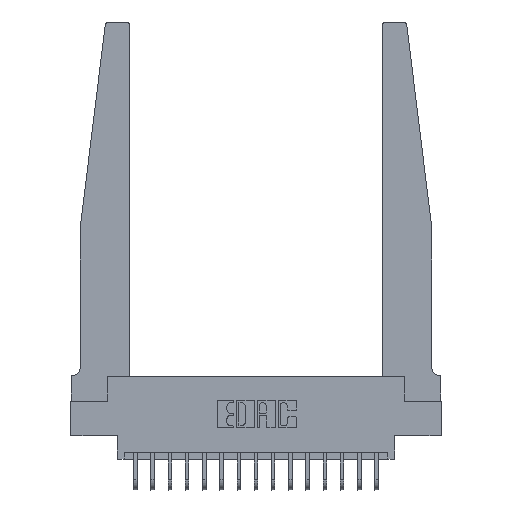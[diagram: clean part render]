
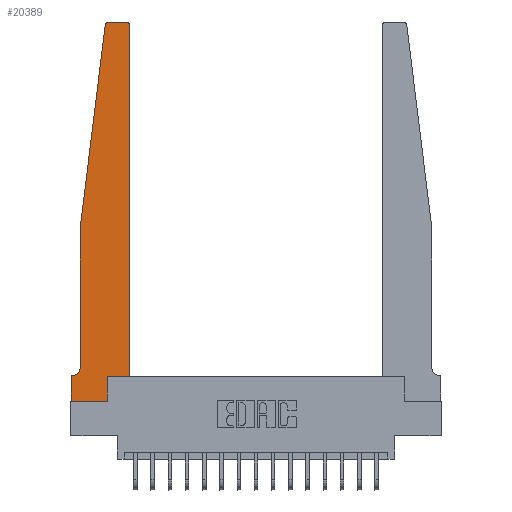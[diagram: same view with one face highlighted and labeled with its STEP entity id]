
A CAD part, top view. The second image highlights one B-rep face of the part: STEP entity #20389.
In plain terms, the highlighted planar face has unit normal (0, 0, 1).
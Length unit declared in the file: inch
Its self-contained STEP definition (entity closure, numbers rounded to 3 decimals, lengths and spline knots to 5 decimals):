
#26 = EDGE_CURVE ( 'NONE', #13548, #12404, #19728, .T. ) ;
#294 = VECTOR ( 'NONE', #3807, 39.37008 ) ;
#402 = LINE ( 'NONE', #8385, #9618 ) ;
#547 = VECTOR ( 'NONE', #7833, 39.37008 ) ;
#580 = AXIS2_PLACEMENT_3D ( 'NONE', #13098, #8031, #12697 ) ;
#652 = LINE ( 'NONE', #5311, #12384 ) ;
#722 = ORIENTED_EDGE ( 'NONE', *, *, #2862, .T. ) ;
#747 = DIRECTION ( 'NONE',  ( 0., 0., 1. ) ) ;
#812 = CARTESIAN_POINT ( 'NONE',  ( 0.065, 0.2375, 0.37 ) ) ;
#881 = VECTOR ( 'NONE', #3115, 39.37008 ) ;
#893 = CARTESIAN_POINT ( 'NONE',  ( 0.27653, 2.72, 0.37 ) ) ;
#1056 = CARTESIAN_POINT ( 'NONE',  ( 0.2605, 0.18, 0.37 ) ) ;
#1185 = VECTOR ( 'NONE', #11797, 39.37008 ) ;
#1260 = CARTESIAN_POINT ( 'NONE',  ( 0.425, 0.18, 0.37 ) ) ;
#1455 = ORIENTED_EDGE ( 'NONE', *, *, #6493, .T. ) ;
#1511 = VERTEX_POINT ( 'NONE', #7853 ) ;
#1911 = LINE ( 'NONE', #9801, #547 ) ;
#1984 = EDGE_CURVE ( 'NONE', #12404, #7132, #652, .T. ) ;
#2103 = VERTEX_POINT ( 'NONE', #12172 ) ;
#2400 = CARTESIAN_POINT ( 'NONE',  ( 0.015, 0.2375, 0.37 ) ) ;
#2664 = CARTESIAN_POINT ( 'NONE',  ( 0.425, 2.72, 0.37 ) ) ;
#2816 = EDGE_CURVE ( 'NONE', #4783, #9039, #6826, .T. ) ;
#2862 = EDGE_CURVE ( 'NONE', #7132, #19450, #402, .T. ) ;
#2915 = CARTESIAN_POINT ( 'NONE',  ( 0., 0., 0.37 ) ) ;
#3115 = DIRECTION ( 'NONE',  ( 1., 0., 0. ) ) ;
#3807 = DIRECTION ( 'NONE',  ( -1., 0., 0. ) ) ;
#4257 = ORIENTED_EDGE ( 'NONE', *, *, #26, .T. ) ;
#4278 = VECTOR ( 'NONE', #16283, 39.37008 ) ;
#4649 = VERTEX_POINT ( 'NONE', #19947 ) ;
#4783 = VERTEX_POINT ( 'NONE', #18880 ) ;
#5241 = LINE ( 'NONE', #16152, #19628 ) ;
#5311 = CARTESIAN_POINT ( 'NONE',  ( 0.425, 0.18, 0.37 ) ) ;
#5462 = CARTESIAN_POINT ( 'NONE',  ( 0.2605, 0.18, 0.37 ) ) ;
#5752 = ORIENTED_EDGE ( 'NONE', *, *, #13202, .T. ) ;
#5851 = AXIS2_PLACEMENT_3D ( 'NONE', #14955, #747, #11846 ) ;
#5919 = CIRCLE ( 'NONE', #19534, 0.05 ) ;
#6171 = CARTESIAN_POINT ( 'NONE',  ( 0., 0., 0.37 ) ) ;
#6215 = EDGE_CURVE ( 'NONE', #4649, #16730, #15127, .T. ) ;
#6493 = EDGE_CURVE ( 'NONE', #1511, #10956, #1911, .T. ) ;
#6805 = DIRECTION ( 'NONE',  ( -0.122, -0.992, 0. ) ) ;
#6826 = LINE ( 'NONE', #14705, #4278 ) ;
#6971 = FACE_OUTER_BOUND ( 'NONE', #12750, .T. ) ;
#7064 = DIRECTION ( 'NONE',  ( -1., 0., 0. ) ) ;
#7132 = VERTEX_POINT ( 'NONE', #1260 ) ;
#7482 = EDGE_CURVE ( 'NONE', #19450, #2103, #13494, .T. ) ;
#7833 = DIRECTION ( 'NONE',  ( 0., -1., 0. ) ) ;
#7853 = CARTESIAN_POINT ( 'NONE',  ( 0., 0.1875, 0.37 ) ) ;
#8028 = ORIENTED_EDGE ( 'NONE', *, *, #7482, .T. ) ;
#8031 = DIRECTION ( 'NONE',  ( 0., 0., 1. ) ) ;
#8385 = CARTESIAN_POINT ( 'NONE',  ( 0.425, 0.18, 0.37 ) ) ;
#8632 = PLANE ( 'NONE',  #5851 ) ;
#8839 = ORIENTED_EDGE ( 'NONE', *, *, #2816, .T. ) ;
#9039 = VERTEX_POINT ( 'NONE', #812 ) ;
#9146 = ORIENTED_EDGE ( 'NONE', *, *, #10319, .T. ) ;
#9498 = CARTESIAN_POINT ( 'NONE',  ( 0.2605, 0., 0.37 ) ) ;
#9618 = VECTOR ( 'NONE', #15972, 39.37008 ) ;
#9659 = CARTESIAN_POINT ( 'NONE',  ( 0.015, 0.1875, 0.37 ) ) ;
#9801 = CARTESIAN_POINT ( 'NONE',  ( 0., 0., 0.37 ) ) ;
#10319 = EDGE_CURVE ( 'NONE', #9039, #18709, #5919, .T. ) ;
#10409 = DIRECTION ( 'NONE',  ( -1., 0., 0. ) ) ;
#10610 = LINE ( 'NONE', #19765, #16616 ) ;
#10771 = EDGE_CURVE ( 'NONE', #18709, #1511, #15028, .T. ) ;
#10956 = VERTEX_POINT ( 'NONE', #6171 ) ;
#11797 = DIRECTION ( 'NONE',  ( 0., 1., 0. ) ) ;
#11846 = DIRECTION ( 'NONE',  ( 1., 0., 0. ) ) ;
#12172 = CARTESIAN_POINT ( 'NONE',  ( 0.395, 2.75, 0.37 ) ) ;
#12341 = ORIENTED_EDGE ( 'NONE', *, *, #15403, .T. ) ;
#12384 = VECTOR ( 'NONE', #17986, 39.37008 ) ;
#12404 = VERTEX_POINT ( 'NONE', #1056 ) ;
#12453 = LINE ( 'NONE', #2915, #881 ) ;
#12697 = DIRECTION ( 'NONE',  ( 1., 0., 0. ) ) ;
#12750 = EDGE_LOOP ( 'NONE', ( #12341, #13940, #5752, #8839, #9146, #12940, #1455, #15130, #4257, #16231, #722, #8028 ) ) ;
#12940 = ORIENTED_EDGE ( 'NONE', *, *, #10771, .T. ) ;
#13098 = CARTESIAN_POINT ( 'NONE',  ( 0.395, 2.72, 0.37 ) ) ;
#13129 = DIRECTION ( 'NONE',  ( 0., 0., 1. ) ) ;
#13202 = EDGE_CURVE ( 'NONE', #16730, #4783, #5241, .T. ) ;
#13494 = CIRCLE ( 'NONE', #580, 0.03 ) ;
#13548 = VERTEX_POINT ( 'NONE', #9498 ) ;
#13734 = CARTESIAN_POINT ( 'NONE',  ( 0.24675, 2.72367, 0.37 ) ) ;
#13940 = ORIENTED_EDGE ( 'NONE', *, *, #6215, .T. ) ;
#14453 = AXIS2_PLACEMENT_3D ( 'NONE', #893, #13129, #19611 ) ;
#14705 = CARTESIAN_POINT ( 'NONE',  ( 0.065, 1.25, 0.37 ) ) ;
#14955 = CARTESIAN_POINT ( 'NONE',  ( 0., 0.1875, 0.37 ) ) ;
#15028 = LINE ( 'NONE', #19842, #294 ) ;
#15127 = CIRCLE ( 'NONE', #14453, 0.03 ) ;
#15130 = ORIENTED_EDGE ( 'NONE', *, *, #20408, .T. ) ;
#15403 = EDGE_CURVE ( 'NONE', #2103, #4649, #10610, .T. ) ;
#15972 = DIRECTION ( 'NONE',  ( 0., 1., 0. ) ) ;
#16152 = CARTESIAN_POINT ( 'NONE',  ( 0.065, 1.25, 0.37 ) ) ;
#16231 = ORIENTED_EDGE ( 'NONE', *, *, #1984, .T. ) ;
#16283 = DIRECTION ( 'NONE',  ( 0., -1., 0. ) ) ;
#16616 = VECTOR ( 'NONE', #10409, 39.37008 ) ;
#16730 = VERTEX_POINT ( 'NONE', #13734 ) ;
#17871 = DIRECTION ( 'NONE',  ( 0., 0., -1. ) ) ;
#17986 = DIRECTION ( 'NONE',  ( 1., 0., 0. ) ) ;
#18709 = VERTEX_POINT ( 'NONE', #9659 ) ;
#18880 = CARTESIAN_POINT ( 'NONE',  ( 0.065, 1.25, 0.37 ) ) ;
#19450 = VERTEX_POINT ( 'NONE', #2664 ) ;
#19534 = AXIS2_PLACEMENT_3D ( 'NONE', #2400, #17871, #7064 ) ;
#19611 = DIRECTION ( 'NONE',  ( 1., 0., 0. ) ) ;
#19628 = VECTOR ( 'NONE', #6805, 39.37008 ) ;
#19728 = LINE ( 'NONE', #5462, #1185 ) ;
#19765 = CARTESIAN_POINT ( 'NONE',  ( 0.25, 2.75, 0.37 ) ) ;
#19842 = CARTESIAN_POINT ( 'NONE',  ( 0.065, 0.1875, 0.37 ) ) ;
#19947 = CARTESIAN_POINT ( 'NONE',  ( 0.27653, 2.75, 0.37 ) ) ;
#20389 = ADVANCED_FACE ( 'NONE', ( #6971 ), #8632, .T. ) ;
#20408 = EDGE_CURVE ( 'NONE', #10956, #13548, #12453, .T. ) ;
